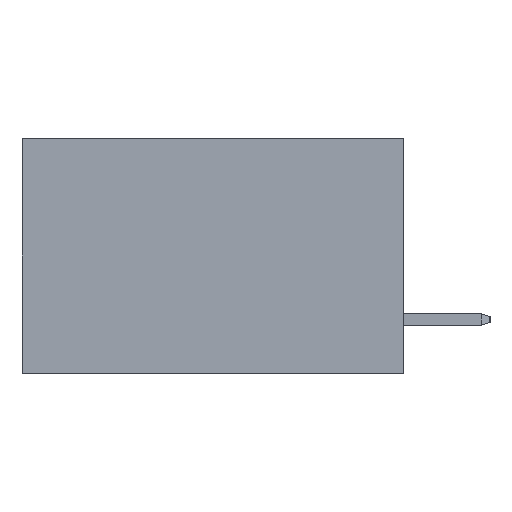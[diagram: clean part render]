
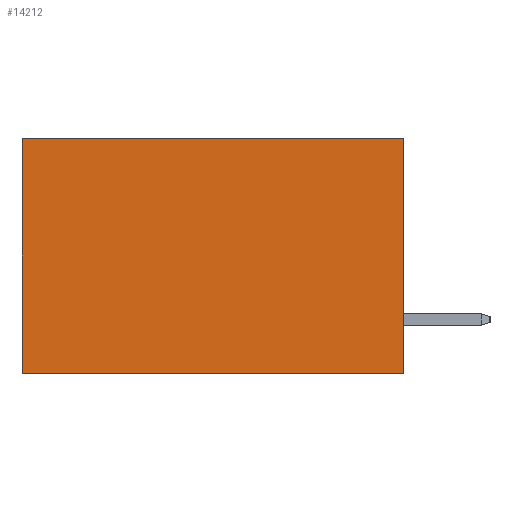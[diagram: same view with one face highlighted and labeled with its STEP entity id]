
A CAD part, left-side view. The second image highlights one B-rep face of the part: STEP entity #14212.
In plain terms, the highlighted planar face has unit normal (-1, 0, 0).
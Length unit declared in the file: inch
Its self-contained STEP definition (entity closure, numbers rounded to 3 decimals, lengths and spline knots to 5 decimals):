
#430 = VERTEX_POINT ( 'NONE', #2256 ) ;
#435 = CARTESIAN_POINT ( 'NONE',  ( 0.2875, 0., 0. ) ) ;
#699 = CARTESIAN_POINT ( 'NONE',  ( 0.2875, 0., 0. ) ) ;
#725 = VERTEX_POINT ( 'NONE', #6226 ) ;
#1025 = VECTOR ( 'NONE', #7307, 39.37008 ) ;
#1306 = ORIENTED_EDGE ( 'NONE', *, *, #14919, .F. ) ;
#2256 = CARTESIAN_POINT ( 'NONE',  ( 0.2875, 0., -0.37 ) ) ;
#2853 = DIRECTION ( 'NONE',  ( 0., 1., 0. ) ) ;
#3206 = EDGE_CURVE ( 'NONE', #3275, #725, #4523, .T. ) ;
#3275 = VERTEX_POINT ( 'NONE', #10267 ) ;
#3917 = FACE_OUTER_BOUND ( 'NONE', #14341, .T. ) ;
#3957 = CARTESIAN_POINT ( 'NONE',  ( 0.2875, 0., -0.37 ) ) ;
#4515 = DIRECTION ( 'NONE',  ( 1., 0., 0. ) ) ;
#4523 = LINE ( 'NONE', #9837, #1025 ) ;
#4960 = VECTOR ( 'NONE', #2853, 39.37008 ) ;
#4972 = AXIS2_PLACEMENT_3D ( 'NONE', #8516, #4515, #9995 ) ;
#6226 = CARTESIAN_POINT ( 'NONE',  ( 0.2875, 0.6, -0.37 ) ) ;
#7225 = VECTOR ( 'NONE', #14085, 39.37008 ) ;
#7307 = DIRECTION ( 'NONE',  ( 0., 0., -1. ) ) ;
#8105 = PLANE ( 'NONE',  #4972 ) ;
#8493 = LINE ( 'NONE', #10951, #4960 ) ;
#8516 = CARTESIAN_POINT ( 'NONE',  ( 0.2875, 0., 0. ) ) ;
#8797 = ORIENTED_EDGE ( 'NONE', *, *, #9954, .F. ) ;
#9837 = CARTESIAN_POINT ( 'NONE',  ( 0.2875, 0.6, 0. ) ) ;
#9954 = EDGE_CURVE ( 'NONE', #17158, #430, #15568, .T. ) ;
#9995 = DIRECTION ( 'NONE',  ( 0., 0., -1. ) ) ;
#10267 = CARTESIAN_POINT ( 'NONE',  ( 0.2875, 0.6, 0. ) ) ;
#10951 = CARTESIAN_POINT ( 'NONE',  ( 0.2875, 0., 0. ) ) ;
#12019 = ORIENTED_EDGE ( 'NONE', *, *, #13370, .T. ) ;
#13355 = ORIENTED_EDGE ( 'NONE', *, *, #3206, .T. ) ;
#13360 = VECTOR ( 'NONE', #15961, 39.37008 ) ;
#13370 = EDGE_CURVE ( 'NONE', #17158, #3275, #8493, .T. ) ;
#14085 = DIRECTION ( 'NONE',  ( 0., 0., -1. ) ) ;
#14212 = ADVANCED_FACE ( 'NONE', ( #3917 ), #8105, .F. ) ;
#14341 = EDGE_LOOP ( 'NONE', ( #13355, #1306, #8797, #12019 ) ) ;
#14919 = EDGE_CURVE ( 'NONE', #430, #725, #15789, .T. ) ;
#15568 = LINE ( 'NONE', #699, #7225 ) ;
#15789 = LINE ( 'NONE', #3957, #13360 ) ;
#15961 = DIRECTION ( 'NONE',  ( 0., 1., 0. ) ) ;
#17158 = VERTEX_POINT ( 'NONE', #435 ) ;
